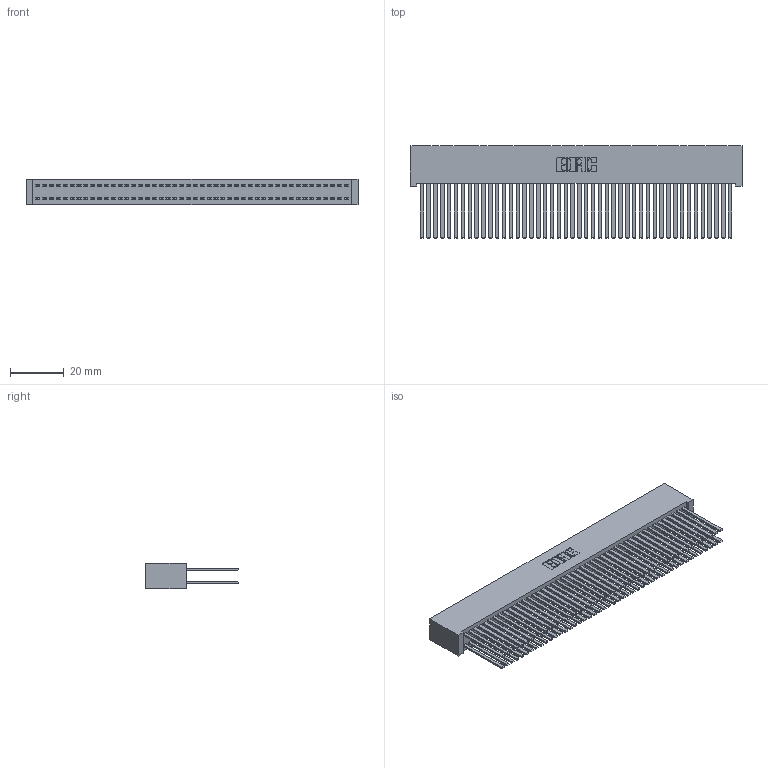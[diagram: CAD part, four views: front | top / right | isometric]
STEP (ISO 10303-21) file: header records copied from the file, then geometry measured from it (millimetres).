
FILE_DESCRIPTION (( 'STEP AP203' ), '1' );
FILE_NAME ('392-092-544-201.STEP', '2019-10-09T18:57:58', ( '' ), ( '' ), 'SwSTEP 2.0', 'SolidWorks 2016', '' );
FILE_SCHEMA (( 'CONFIG_CONTROL_DESIGN' ));
Length unit declared in the file: inch
Products named in the file (3): 342 Part_Lugless; 345-292-001_345-293-144; 392-092-544-201
Assembly tree (93 placements, depth 2):
  392-092-544-201
    342 Part_Lugless
    345-292-001_345-293-144  x92
Bounding box: 123.09 x 34.3 x 9.4 mm (x, y, z)
Volume: 12807.6 mm3; surface area: 24963.9 mm2
Topology: 93 solids, 93 shells, 4334 faces, 12879 edges, 8462 vertices
Faces by surface type: plane 3006, cylinder 1328
Entity records: 28483 total; most frequent: CARTESIAN_POINT 4710, ORIENTED_EDGE 4646, DIRECTION 4007, EDGE_CURVE 2323, LINE 2207, VECTOR 2207, VERTEX_POINT 1546, AXIS2_PLACEMENT_3D 900
